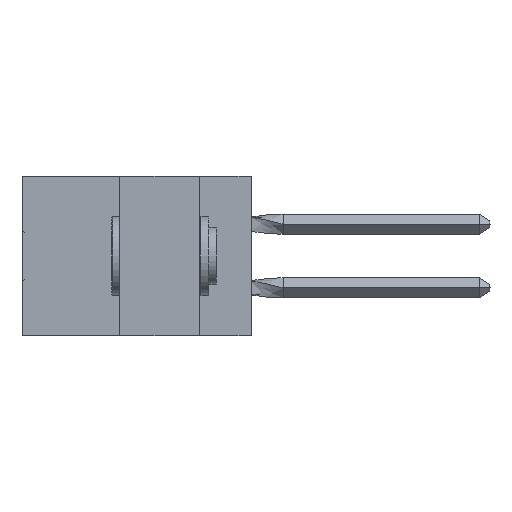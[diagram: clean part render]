
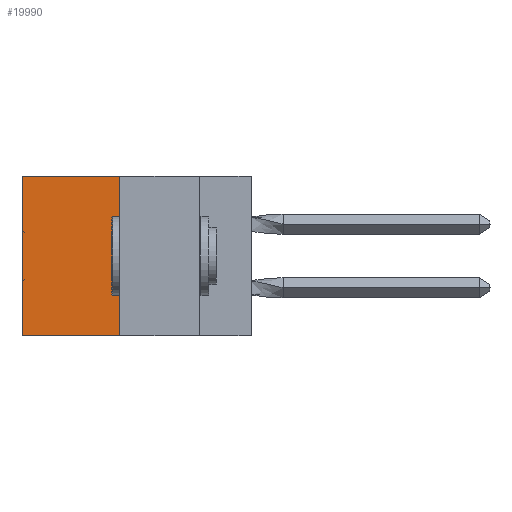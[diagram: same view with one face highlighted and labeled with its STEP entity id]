
A CAD part, left-side view. The second image highlights one B-rep face of the part: STEP entity #19990.
In plain terms, the highlighted planar face has unit normal (-1, 0, 0).
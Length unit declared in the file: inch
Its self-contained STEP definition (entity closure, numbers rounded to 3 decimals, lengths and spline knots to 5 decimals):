
#4184 = CARTESIAN_POINT ( 'NONE',  ( 0.305, 0.72, -0.5 ) ) ;
#4585 = VECTOR ( 'NONE', #6344, 39.37008 ) ;
#5438 = CARTESIAN_POINT ( 'NONE',  ( 0.305, 0.72, -0.5 ) ) ;
#5975 = CARTESIAN_POINT ( 'NONE',  ( 0.305, 0.413, -0.5 ) ) ;
#6344 = DIRECTION ( 'NONE',  ( 0., 1., 0. ) ) ;
#7300 = EDGE_CURVE ( 'NONE', #47243, #49219, #18886, .T. ) ;
#8040 = EDGE_LOOP ( 'NONE', ( #19861, #34539, #48883, #17816 ) ) ;
#11106 = VERTEX_POINT ( 'NONE', #34384 ) ;
#11689 = VECTOR ( 'NONE', #42351, 39.37008 ) ;
#12575 = CARTESIAN_POINT ( 'NONE',  ( 0.305, 0.413, -0.5 ) ) ;
#14368 = EDGE_CURVE ( 'NONE', #33730, #49219, #17767, .T. ) ;
#16020 = DIRECTION ( 'NONE',  ( 0., 0., -1. ) ) ;
#16057 = CARTESIAN_POINT ( 'NONE',  ( 0.305, 0.413, 0. ) ) ;
#17767 = LINE ( 'NONE', #4184, #49601 ) ;
#17816 = ORIENTED_EDGE ( 'NONE', *, *, #50826, .T. ) ;
#18886 = LINE ( 'NONE', #5975, #4585 ) ;
#19861 = ORIENTED_EDGE ( 'NONE', *, *, #14368, .T. ) ;
#19990 = ADVANCED_FACE ( 'NONE', ( #28344 ), #20569, .F. ) ;
#20569 = PLANE ( 'NONE',  #24054 ) ;
#21421 = LINE ( 'NONE', #12575, #11689 ) ;
#24054 = AXIS2_PLACEMENT_3D ( 'NONE', #53037, #28214, #16020 ) ;
#28214 = DIRECTION ( 'NONE',  ( 1., 0., 0. ) ) ;
#28242 = DIRECTION ( 'NONE',  ( 0., 1., 0. ) ) ;
#28344 = FACE_OUTER_BOUND ( 'NONE', #8040, .T. ) ;
#29311 = DIRECTION ( 'NONE',  ( 0., 0., -1. ) ) ;
#32290 = EDGE_CURVE ( 'NONE', #11106, #47243, #21421, .T. ) ;
#33730 = VERTEX_POINT ( 'NONE', #46399 ) ;
#34384 = CARTESIAN_POINT ( 'NONE',  ( 0.305, 0.413, 0. ) ) ;
#34539 = ORIENTED_EDGE ( 'NONE', *, *, #7300, .F. ) ;
#36259 = VECTOR ( 'NONE', #28242, 39.37008 ) ;
#39463 = LINE ( 'NONE', #16057, #36259 ) ;
#42351 = DIRECTION ( 'NONE',  ( 0., 0., -1. ) ) ;
#44542 = CARTESIAN_POINT ( 'NONE',  ( 0.305, 0.413, -0.5 ) ) ;
#46399 = CARTESIAN_POINT ( 'NONE',  ( 0.305, 0.72, 0. ) ) ;
#47243 = VERTEX_POINT ( 'NONE', #44542 ) ;
#48883 = ORIENTED_EDGE ( 'NONE', *, *, #32290, .F. ) ;
#49219 = VERTEX_POINT ( 'NONE', #5438 ) ;
#49601 = VECTOR ( 'NONE', #29311, 39.37008 ) ;
#50826 = EDGE_CURVE ( 'NONE', #11106, #33730, #39463, .T. ) ;
#53037 = CARTESIAN_POINT ( 'NONE',  ( 0.305, 0.413, -0.5 ) ) ;
